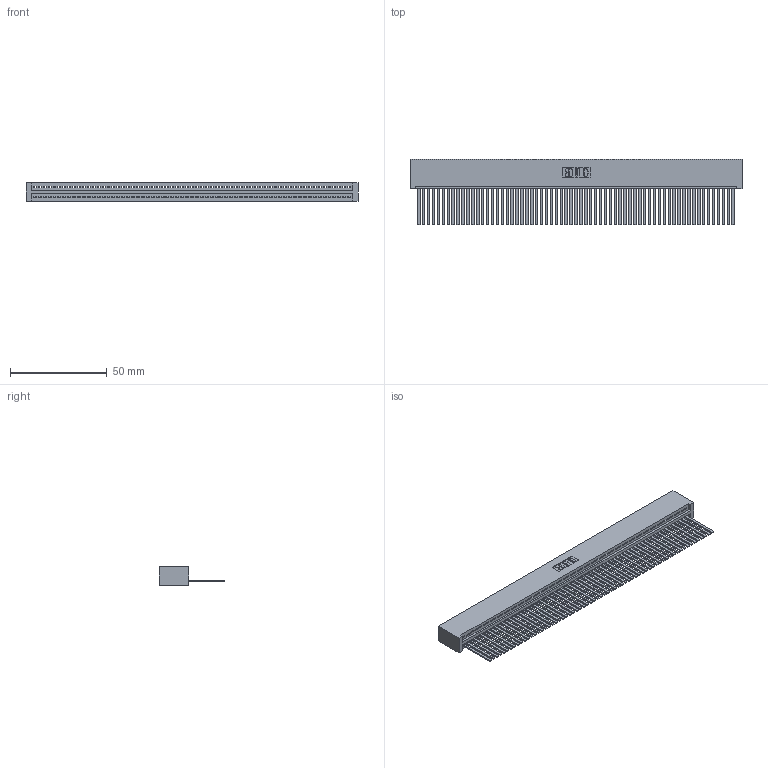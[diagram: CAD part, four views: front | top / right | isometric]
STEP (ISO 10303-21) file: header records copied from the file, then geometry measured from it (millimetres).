
FILE_DESCRIPTION (( 'STEP AP203' ), '1' );
FILE_NAME ('345-065-544-101.STEP', '2019-10-11T19:00:11', ( '' ), ( '' ), 'SwSTEP 2.0', 'SolidWorks 2016', '' );
FILE_SCHEMA (( 'CONFIG_CONTROL_DESIGN' ));
Length unit declared in the file: inch
Products named in the file (3): 345 Part_No Mounting Lugs; 345-065-544-101; 345-292-001_345-293-144
Assembly tree (66 placements, depth 2):
  345-065-544-101
    345 Part_No Mounting Lugs
    345-292-001_345-293-144  x65
Bounding box: 171.7 x 33.96 x 9.4 mm (x, y, z)
Volume: 17834.2 mm3; surface area: 26462.7 mm2
Topology: 66 solids, 66 shells, 3498 faces, 10587 edges, 6970 vertices
Faces by surface type: plane 2416, cylinder 1082
Entity records: 45363 total; most frequent: CARTESIAN_POINT 7863, ORIENTED_EDGE 7862, DIRECTION 6825, EDGE_CURVE 3931, VECTOR 3551, LINE 3551, VERTEX_POINT 2618, AXIS2_PLACEMENT_3D 1637
